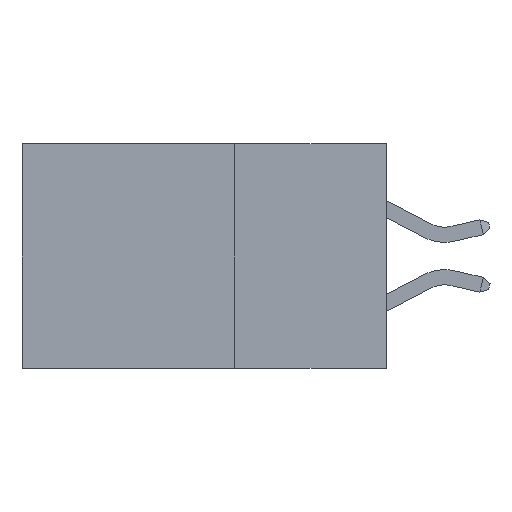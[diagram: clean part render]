
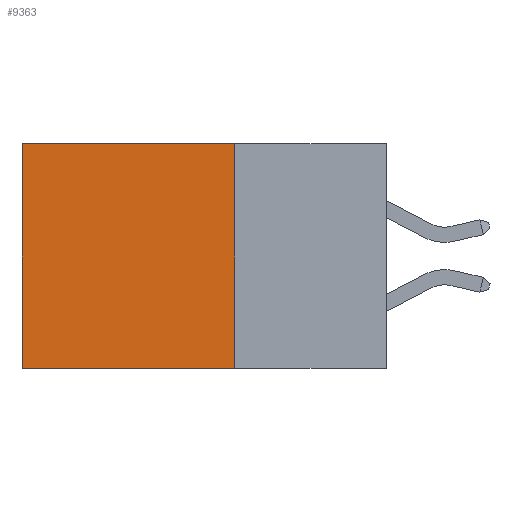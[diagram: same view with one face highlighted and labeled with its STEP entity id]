
A CAD part, left-side view. The second image highlights one B-rep face of the part: STEP entity #9363.
In plain terms, the highlighted planar face has unit normal (-1, 0, 0).
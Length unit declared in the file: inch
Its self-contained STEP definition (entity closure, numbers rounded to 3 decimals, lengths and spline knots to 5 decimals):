
#1587 = EDGE_CURVE ( 'NONE', #10610, #12571, #10724, .T. ) ;
#1717 = VERTEX_POINT ( 'NONE', #6852 ) ;
#2068 = CARTESIAN_POINT ( 'NONE',  ( 0.2615, 0.25, 0. ) ) ;
#2357 = DIRECTION ( 'NONE',  ( 0., 0., -1. ) ) ;
#2379 = CARTESIAN_POINT ( 'NONE',  ( 0.2615, 0.6, -0.37 ) ) ;
#3574 = VERTEX_POINT ( 'NONE', #20316 ) ;
#3676 = ORIENTED_EDGE ( 'NONE', *, *, #10537, .T. ) ;
#4887 = EDGE_LOOP ( 'NONE', ( #3676, #24078, #17150, #20815 ) ) ;
#6852 = CARTESIAN_POINT ( 'NONE',  ( 0.2615, 0.6, 0. ) ) ;
#8004 = VECTOR ( 'NONE', #22834, 39.37008 ) ;
#9363 = ADVANCED_FACE ( 'NONE', ( #15783 ), #14292, .F. ) ;
#9761 = DIRECTION ( 'NONE',  ( 0., 0., -1. ) ) ;
#10537 = EDGE_CURVE ( 'NONE', #1717, #3574, #18642, .T. ) ;
#10610 = VERTEX_POINT ( 'NONE', #2068 ) ;
#10724 = LINE ( 'NONE', #20755, #11929 ) ;
#11929 = VECTOR ( 'NONE', #9761, 39.37008 ) ;
#12571 = VERTEX_POINT ( 'NONE', #14723 ) ;
#13150 = LINE ( 'NONE', #14471, #22612 ) ;
#14214 = DIRECTION ( 'NONE',  ( 0., 0., -1. ) ) ;
#14234 = DIRECTION ( 'NONE',  ( 1., 0., 0. ) ) ;
#14265 = CARTESIAN_POINT ( 'NONE',  ( 0.2615, 0.25, -0.37 ) ) ;
#14292 = PLANE ( 'NONE',  #21507 ) ;
#14471 = CARTESIAN_POINT ( 'NONE',  ( 0.2615, 0.25, 0. ) ) ;
#14723 = CARTESIAN_POINT ( 'NONE',  ( 0.2615, 0.25, -0.37 ) ) ;
#15783 = FACE_OUTER_BOUND ( 'NONE', #4887, .T. ) ;
#16354 = DIRECTION ( 'NONE',  ( 0., 1., 0. ) ) ;
#16446 = EDGE_CURVE ( 'NONE', #10610, #1717, #13150, .T. ) ;
#17150 = ORIENTED_EDGE ( 'NONE', *, *, #1587, .F. ) ;
#17286 = EDGE_CURVE ( 'NONE', #12571, #3574, #18125, .T. ) ;
#18125 = LINE ( 'NONE', #20923, #8004 ) ;
#18642 = LINE ( 'NONE', #2379, #24254 ) ;
#20316 = CARTESIAN_POINT ( 'NONE',  ( 0.2615, 0.6, -0.37 ) ) ;
#20755 = CARTESIAN_POINT ( 'NONE',  ( 0.2615, 0.25, -0.37 ) ) ;
#20815 = ORIENTED_EDGE ( 'NONE', *, *, #16446, .T. ) ;
#20923 = CARTESIAN_POINT ( 'NONE',  ( 0.2615, 0.25, -0.37 ) ) ;
#21507 = AXIS2_PLACEMENT_3D ( 'NONE', #14265, #14234, #14214 ) ;
#22612 = VECTOR ( 'NONE', #16354, 39.37008 ) ;
#22834 = DIRECTION ( 'NONE',  ( 0., 1., 0. ) ) ;
#24078 = ORIENTED_EDGE ( 'NONE', *, *, #17286, .F. ) ;
#24254 = VECTOR ( 'NONE', #2357, 39.37008 ) ;
